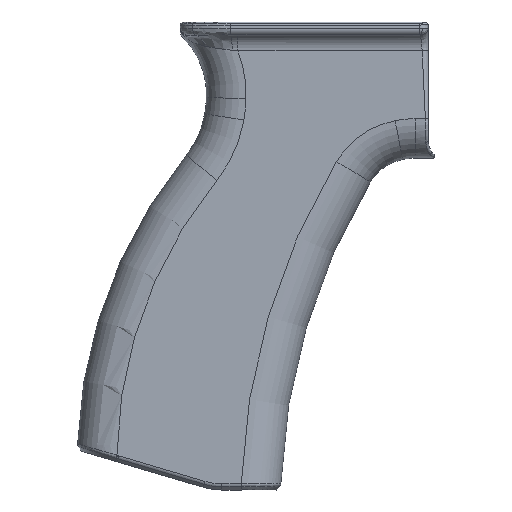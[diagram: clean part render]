
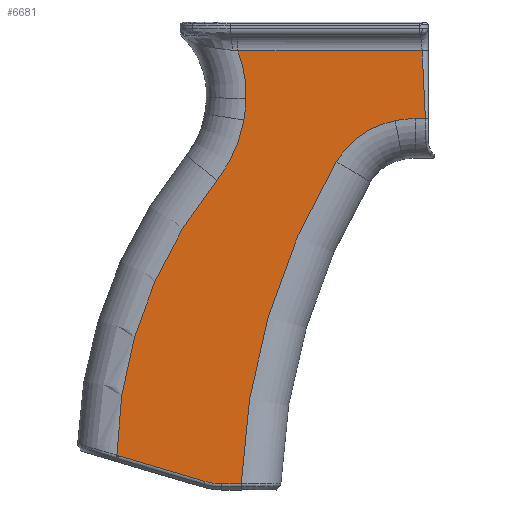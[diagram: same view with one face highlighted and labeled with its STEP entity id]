
A CAD part, front view. The second image highlights one B-rep face of the part: STEP entity #6681.
In plain terms, the highlighted planar face has unit normal (0, -1, 0).
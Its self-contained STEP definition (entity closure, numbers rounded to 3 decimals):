
#346=PLANE('',#7162);
#403=FACE_OUTER_BOUND('',#861,.T.);
#861=EDGE_LOOP('',(#4413,#4414,#4415,#4416,#4417,#4418,#4419,#4420,#4421,
#4422,#4423,#4424,#4425,#4426,#4427,#4428,#4429));
#1325=B_SPLINE_CURVE_WITH_KNOTS('',3,(#9305,#9306,#9307,#9308),
 .UNSPECIFIED.,.F.,.F.,(4,4),(0.,0.013),.UNSPECIFIED.);
#1326=B_SPLINE_CURVE_WITH_KNOTS('',3,(#9310,#9311,#9312,#9313),
 .UNSPECIFIED.,.F.,.F.,(4,4),(0.,0.028),.UNSPECIFIED.);
#1327=B_SPLINE_CURVE_WITH_KNOTS('',3,(#9321,#9322,#9323,#9324),
 .UNSPECIFIED.,.F.,.F.,(4,4),(0.,0.003),.UNSPECIFIED.);
#1328=B_SPLINE_CURVE_WITH_KNOTS('',3,(#9326,#9327,#9328,#9329),
 .UNSPECIFIED.,.F.,.F.,(4,4),(0.,0.001),.UNSPECIFIED.);
#1329=B_SPLINE_CURVE_WITH_KNOTS('',3,(#9339,#9340,#9341,#9342),
 .UNSPECIFIED.,.F.,.F.,(4,4),(5.216,6.761),
 .UNSPECIFIED.);
#1766=CIRCLE('',#7163,29.);
#1767=CIRCLE('',#7164,101.565);
#1768=CIRCLE('',#7165,13.586);
#1769=CIRCLE('',#7166,152.175);
#1770=CIRCLE('',#7167,20.);
#1771=CIRCLE('',#7168,24.);
#1772=CIRCLE('',#7169,27.);
#1773=CIRCLE('',#7170,41.022);
#2141=LINE('',#9315,#2406);
#2142=LINE('',#9319,#2407);
#2143=LINE('',#9337,#2408);
#2144=LINE('',#9344,#2409);
#2406=VECTOR('',#7804,10.);
#2407=VECTOR('',#7807,10.);
#2408=VECTOR('',#7814,10.);
#2409=VECTOR('',#7815,4.);
#2681=VERTEX_POINT('',#9299);
#2682=VERTEX_POINT('',#9300);
#2683=VERTEX_POINT('',#9302);
#2684=VERTEX_POINT('',#9304);
#2685=VERTEX_POINT('',#9309);
#2686=VERTEX_POINT('',#9314);
#2687=VERTEX_POINT('',#9316);
#2688=VERTEX_POINT('',#9318);
#2689=VERTEX_POINT('',#9320);
#2690=VERTEX_POINT('',#9325);
#2691=VERTEX_POINT('',#9330);
#2692=VERTEX_POINT('',#9332);
#2693=VERTEX_POINT('',#9334);
#2694=VERTEX_POINT('',#9336);
#2695=VERTEX_POINT('',#9338);
#2696=VERTEX_POINT('',#9343);
#2697=VERTEX_POINT('',#9345);
#3323=EDGE_CURVE('',#2681,#2682,#1766,.T.);
#3324=EDGE_CURVE('',#2682,#2683,#1767,.T.);
#3325=EDGE_CURVE('',#2683,#2684,#1325,.T.);
#3326=EDGE_CURVE('',#2684,#2685,#1326,.T.);
#3327=EDGE_CURVE('',#2685,#2686,#2141,.T.);
#3328=EDGE_CURVE('',#2686,#2687,#1768,.T.);
#3329=EDGE_CURVE('',#2687,#2688,#2142,.T.);
#3330=EDGE_CURVE('',#2688,#2689,#1327,.T.);
#3331=EDGE_CURVE('',#2689,#2690,#1328,.T.);
#3332=EDGE_CURVE('',#2690,#2691,#1769,.T.);
#3333=EDGE_CURVE('',#2691,#2692,#1770,.T.);
#3334=EDGE_CURVE('',#2692,#2693,#1771,.T.);
#3335=EDGE_CURVE('',#2693,#2694,#2143,.T.);
#3336=EDGE_CURVE('',#2694,#2695,#1329,.T.);
#3337=EDGE_CURVE('',#2695,#2696,#2144,.T.);
#3338=EDGE_CURVE('',#2696,#2697,#1772,.T.);
#3339=EDGE_CURVE('',#2697,#2681,#1773,.T.);
#4413=ORIENTED_EDGE('',*,*,#3323,.T.);
#4414=ORIENTED_EDGE('',*,*,#3324,.T.);
#4415=ORIENTED_EDGE('',*,*,#3325,.T.);
#4416=ORIENTED_EDGE('',*,*,#3326,.T.);
#4417=ORIENTED_EDGE('',*,*,#3327,.T.);
#4418=ORIENTED_EDGE('',*,*,#3328,.T.);
#4419=ORIENTED_EDGE('',*,*,#3329,.T.);
#4420=ORIENTED_EDGE('',*,*,#3330,.T.);
#4421=ORIENTED_EDGE('',*,*,#3331,.T.);
#4422=ORIENTED_EDGE('',*,*,#3332,.T.);
#4423=ORIENTED_EDGE('',*,*,#3333,.T.);
#4424=ORIENTED_EDGE('',*,*,#3334,.T.);
#4425=ORIENTED_EDGE('',*,*,#3335,.T.);
#4426=ORIENTED_EDGE('',*,*,#3336,.T.);
#4427=ORIENTED_EDGE('',*,*,#3337,.T.);
#4428=ORIENTED_EDGE('',*,*,#3338,.T.);
#4429=ORIENTED_EDGE('',*,*,#3339,.T.);
#6681=ADVANCED_FACE('',(#403),#346,.F.);
#7162=AXIS2_PLACEMENT_3D('',#9298,#7798,#7799);
#7163=AXIS2_PLACEMENT_3D('',#9301,#7800,#7801);
#7164=AXIS2_PLACEMENT_3D('',#9303,#7802,#7803);
#7165=AXIS2_PLACEMENT_3D('',#9317,#7805,#7806);
#7166=AXIS2_PLACEMENT_3D('',#9331,#7808,#7809);
#7167=AXIS2_PLACEMENT_3D('',#9333,#7810,#7811);
#7168=AXIS2_PLACEMENT_3D('',#9335,#7812,#7813);
#7169=AXIS2_PLACEMENT_3D('',#9346,#7816,#7817);
#7170=AXIS2_PLACEMENT_3D('',#9347,#7818,#7819);
#7798=DIRECTION('center_axis',(0.,1.,0.));
#7799=DIRECTION('ref_axis',(0.,0.,-1.));
#7800=DIRECTION('center_axis',(0.,1.,0.));
#7801=DIRECTION('ref_axis',(0.913,0.,-0.409));
#7802=DIRECTION('center_axis',(0.,-1.,0.));
#7803=DIRECTION('ref_axis',(-0.79,0.,0.613));
#7804=DIRECTION('',(0.959,0.,-0.284));
#7805=DIRECTION('center_axis',(0.,-1.,0.));
#7806=DIRECTION('ref_axis',(-0.144,0.,-0.99));
#7807=DIRECTION('',(1.,0.,0.));
#7808=DIRECTION('center_axis',(0.,1.,0.));
#7809=DIRECTION('ref_axis',(-0.871,0.,0.491));
#7810=DIRECTION('center_axis',(0.,1.,0.));
#7811=DIRECTION('ref_axis',(-0.573,0.,0.819));
#7812=DIRECTION('center_axis',(0.,1.,0.));
#7813=DIRECTION('ref_axis',(-0.095,0.,0.995));
#7814=DIRECTION('',(1.,0.,0.));
#7815=DIRECTION('',(-1.,0.,0.));
#7816=DIRECTION('center_axis',(0.,1.,0.));
#7817=DIRECTION('ref_axis',(0.922,0.,0.388));
#7818=DIRECTION('center_axis',(0.,1.,0.));
#7819=DIRECTION('ref_axis',(0.995,0.,-0.1));
#9298=CARTESIAN_POINT('Origin',(-9.956,-10.6,-6.));
#9299=CARTESIAN_POINT('',(7.166,-10.6,-22.312));
#9300=CARTESIAN_POINT('',(1.031,-10.6,-36.013));
#9301=CARTESIAN_POINT('Origin',(-21.468,-10.6,-17.715));
#9302=CARTESIAN_POINT('',(-21.726,-10.6,-98.572));
#9303=CARTESIAN_POINT('Origin',(79.827,-10.6,-100.095));
#9304=CARTESIAN_POINT('',(-21.599,-10.6,-98.611));
#9305=CARTESIAN_POINT('Ctrl Pts',(-21.726,-10.6,-98.572));
#9306=CARTESIAN_POINT('Ctrl Pts',(-21.684,-10.6,-98.585));
#9307=CARTESIAN_POINT('Ctrl Pts',(-21.642,-10.6,-98.598));
#9308=CARTESIAN_POINT('Ctrl Pts',(-21.599,-10.6,-98.611));
#9309=CARTESIAN_POINT('',(-21.335,-10.6,-98.691));
#9310=CARTESIAN_POINT('Ctrl Pts',(-21.599,-10.6,-98.611));
#9311=CARTESIAN_POINT('Ctrl Pts',(-21.511,-10.6,-98.638));
#9312=CARTESIAN_POINT('Ctrl Pts',(-21.423,-10.6,-98.664));
#9313=CARTESIAN_POINT('Ctrl Pts',(-21.335,-10.6,-98.691));
#9314=CARTESIAN_POINT('',(-1.686,-10.6,-104.519));
#9315=CARTESIAN_POINT('',(-27.009,-10.6,-97.008));
#9316=CARTESIAN_POINT('',(2.178,-10.6,-105.08));
#9317=CARTESIAN_POINT('Origin',(2.178,-10.6,-91.494));
#9318=CARTESIAN_POINT('',(6.55,-10.6,-105.08));
#9319=CARTESIAN_POINT('',(-5.641,-10.6,-105.08));
#9320=CARTESIAN_POINT('',(6.576,-10.6,-105.08));
#9321=CARTESIAN_POINT('Ctrl Pts',(6.55,-10.6,-105.08));
#9322=CARTESIAN_POINT('Ctrl Pts',(6.559,-10.6,-105.08));
#9323=CARTESIAN_POINT('Ctrl Pts',(6.567,-10.6,-105.08));
#9324=CARTESIAN_POINT('Ctrl Pts',(6.576,-10.6,-105.08));
#9325=CARTESIAN_POINT('',(6.591,-10.6,-105.08));
#9326=CARTESIAN_POINT('Ctrl Pts',(6.576,-10.6,-105.08));
#9327=CARTESIAN_POINT('Ctrl Pts',(6.581,-10.6,-105.08));
#9328=CARTESIAN_POINT('Ctrl Pts',(6.586,-10.6,-105.08));
#9329=CARTESIAN_POINT('Ctrl Pts',(6.591,-10.6,-105.08));
#9330=CARTESIAN_POINT('',(28.244,-10.6,-31.771));
#9331=CARTESIAN_POINT('Origin',(158.681,-10.6,-110.152));
#9332=CARTESIAN_POINT('',(41.592,-10.6,-22.436));
#9333=CARTESIAN_POINT('Origin',(45.387,-10.6,-42.073));
#9334=CARTESIAN_POINT('',(46.147,-10.6,-22.));
#9335=CARTESIAN_POINT('Origin',(46.147,-10.6,-46.));
#9336=CARTESIAN_POINT('',(48.471,-10.6,-22.));
#9337=CARTESIAN_POINT('',(-5.898,-10.6,-22.));
#9338=CARTESIAN_POINT('',(47.747,-10.6,-6.583));
#9339=CARTESIAN_POINT('Ctrl Pts',(48.471,-10.6,-22.));
#9340=CARTESIAN_POINT('Ctrl Pts',(48.324,-10.6,-16.852));
#9341=CARTESIAN_POINT('Ctrl Pts',(48.045,-10.6,-11.719));
#9342=CARTESIAN_POINT('Ctrl Pts',(47.747,-10.6,-6.583));
#9343=CARTESIAN_POINT('',(5.829,-10.6,-6.583));
#9344=CARTESIAN_POINT('',(48.701,-10.6,-6.583));
#9345=CARTESIAN_POINT('',(7.649,-10.6,-17.501));
#9346=CARTESIAN_POINT('Origin',(-19.328,-10.6,-16.388));
#9347=CARTESIAN_POINT('Origin',(-33.338,-10.6,-15.81));
